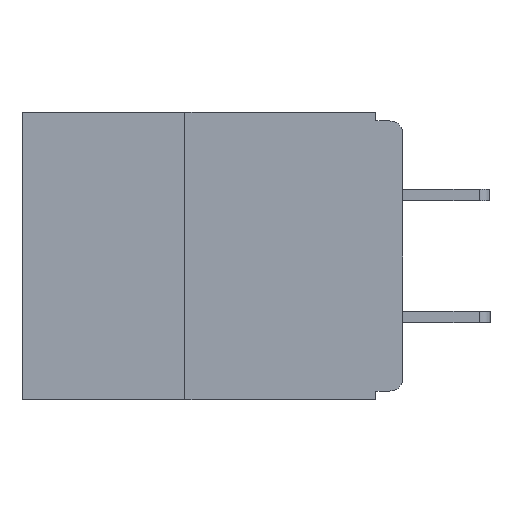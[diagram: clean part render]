
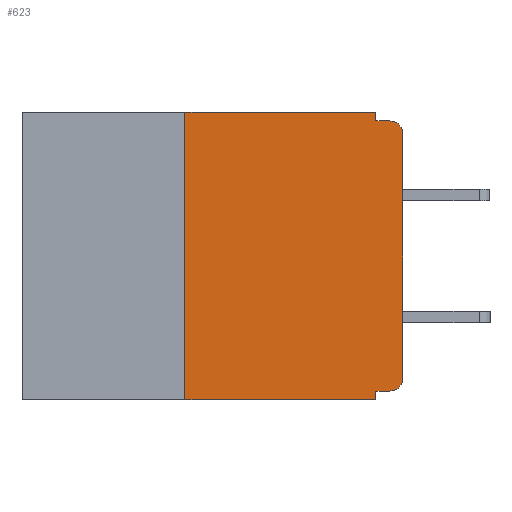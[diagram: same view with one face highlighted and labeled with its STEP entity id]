
A CAD part, left-side view. The second image highlights one B-rep face of the part: STEP entity #623.
In plain terms, the highlighted planar face has unit normal (-1, 0, 0).
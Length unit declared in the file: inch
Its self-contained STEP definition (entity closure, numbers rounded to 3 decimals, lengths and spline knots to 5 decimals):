
#165 = VECTOR ( 'NONE', #5151, 39.37008 ) ;
#623 = ADVANCED_FACE ( 'NONE', ( #1722 ), #1847, .F. ) ;
#680 = VERTEX_POINT ( 'NONE', #10911 ) ;
#707 = EDGE_CURVE ( 'NONE', #10300, #680, #3508, .T. ) ;
#1076 = VERTEX_POINT ( 'NONE', #2092 ) ;
#1090 = LINE ( 'NONE', #6201, #6338 ) ;
#1134 = CARTESIAN_POINT ( 'NONE',  ( 0., 0.015, -0.32 ) ) ;
#1317 = DIRECTION ( 'NONE',  ( 0., 0., 1. ) ) ;
#1501 = AXIS2_PLACEMENT_3D ( 'NONE', #9572, #3896, #10550 ) ;
#1622 = EDGE_CURVE ( 'NONE', #10391, #7050, #1090, .T. ) ;
#1689 = AXIS2_PLACEMENT_3D ( 'NONE', #6691, #3105, #7161 ) ;
#1722 = FACE_OUTER_BOUND ( 'NONE', #4374, .T. ) ;
#1847 = PLANE ( 'NONE',  #7245 ) ;
#1922 = VERTEX_POINT ( 'NONE', #1134 ) ;
#1944 = VERTEX_POINT ( 'NONE', #11863 ) ;
#2092 = CARTESIAN_POINT ( 'NONE',  ( 0., 0.031, -0.32 ) ) ;
#2133 = CARTESIAN_POINT ( 'NONE',  ( 0., 0., 0. ) ) ;
#2451 = DIRECTION ( 'NONE',  ( 0., 0., -1. ) ) ;
#2479 = CARTESIAN_POINT ( 'NONE',  ( 0., 0.015, -0.01 ) ) ;
#2840 = CARTESIAN_POINT ( 'NONE',  ( 0., 0., -0.32 ) ) ;
#2858 = LINE ( 'NONE', #11774, #165 ) ;
#2998 = EDGE_CURVE ( 'NONE', #680, #10391, #6168, .T. ) ;
#3105 = DIRECTION ( 'NONE',  ( -1., 0., 0. ) ) ;
#3428 = CARTESIAN_POINT ( 'NONE',  ( 0., 0.031, -0.33 ) ) ;
#3508 = LINE ( 'NONE', #7914, #8877 ) ;
#3755 = CARTESIAN_POINT ( 'NONE',  ( 0., 0.031, -0.01 ) ) ;
#3896 = DIRECTION ( 'NONE',  ( -1., 0., 0. ) ) ;
#3999 = ORIENTED_EDGE ( 'NONE', *, *, #10636, .T. ) ;
#4087 = EDGE_CURVE ( 'NONE', #1922, #1944, #5985, .T. ) ;
#4145 = DIRECTION ( 'NONE',  ( 1., 0., 0. ) ) ;
#4374 = EDGE_LOOP ( 'NONE', ( #9203, #3999, #7263, #6801, #9052, #5652, #9795, #10099, #8953, #12111 ) ) ;
#4745 = DIRECTION ( 'NONE',  ( 0., 0., -1. ) ) ;
#5121 = VERTEX_POINT ( 'NONE', #2479 ) ;
#5151 = DIRECTION ( 'NONE',  ( 0., -1., 0. ) ) ;
#5175 = CARTESIAN_POINT ( 'NONE',  ( 0., 0., -0.025 ) ) ;
#5315 = CARTESIAN_POINT ( 'NONE',  ( 0., 0.031, 0. ) ) ;
#5644 = EDGE_CURVE ( 'NONE', #7050, #5121, #7927, .T. ) ;
#5652 = ORIENTED_EDGE ( 'NONE', *, *, #707, .F. ) ;
#5707 = CARTESIAN_POINT ( 'NONE',  ( 0., 0.437, 0. ) ) ;
#5985 = CIRCLE ( 'NONE', #1689, 0.015 ) ;
#6168 = LINE ( 'NONE', #11160, #11190 ) ;
#6201 = CARTESIAN_POINT ( 'NONE',  ( 0., 0.031, 0. ) ) ;
#6214 = EDGE_CURVE ( 'NONE', #1944, #10259, #10288, .T. ) ;
#6338 = VECTOR ( 'NONE', #2451, 39.37008 ) ;
#6521 = VECTOR ( 'NONE', #9552, 39.37008 ) ;
#6691 = CARTESIAN_POINT ( 'NONE',  ( 0., 0.015, -0.305 ) ) ;
#6801 = ORIENTED_EDGE ( 'NONE', *, *, #1622, .F. ) ;
#7050 = VERTEX_POINT ( 'NONE', #3755 ) ;
#7161 = DIRECTION ( 'NONE',  ( 0., 0., -1. ) ) ;
#7186 = CARTESIAN_POINT ( 'NONE',  ( 0., 0.031, -0.33 ) ) ;
#7245 = AXIS2_PLACEMENT_3D ( 'NONE', #5707, #4145, #4745 ) ;
#7263 = ORIENTED_EDGE ( 'NONE', *, *, #5644, .F. ) ;
#7585 = EDGE_CURVE ( 'NONE', #1076, #8836, #12124, .T. ) ;
#7763 = VECTOR ( 'NONE', #1317, 39.37008 ) ;
#7836 = DIRECTION ( 'NONE',  ( 0., -1., 0. ) ) ;
#7914 = CARTESIAN_POINT ( 'NONE',  ( 0., 0.25, -0.33 ) ) ;
#7927 = LINE ( 'NONE', #9599, #9553 ) ;
#8482 = EDGE_CURVE ( 'NONE', #1922, #1076, #8754, .T. ) ;
#8754 = LINE ( 'NONE', #2840, #6521 ) ;
#8836 = VERTEX_POINT ( 'NONE', #7186 ) ;
#8877 = VECTOR ( 'NONE', #11070, 39.37008 ) ;
#8953 = ORIENTED_EDGE ( 'NONE', *, *, #8482, .F. ) ;
#9052 = ORIENTED_EDGE ( 'NONE', *, *, #2998, .F. ) ;
#9203 = ORIENTED_EDGE ( 'NONE', *, *, #6214, .T. ) ;
#9437 = CIRCLE ( 'NONE', #1501, 0.015 ) ;
#9552 = DIRECTION ( 'NONE',  ( 0., 1., 0. ) ) ;
#9553 = VECTOR ( 'NONE', #11049, 39.37008 ) ;
#9572 = CARTESIAN_POINT ( 'NONE',  ( 0., 0.015, -0.025 ) ) ;
#9599 = CARTESIAN_POINT ( 'NONE',  ( 0., 0., -0.01 ) ) ;
#9795 = ORIENTED_EDGE ( 'NONE', *, *, #9894, .T. ) ;
#9894 = EDGE_CURVE ( 'NONE', #10300, #8836, #2858, .T. ) ;
#9976 = CARTESIAN_POINT ( 'NONE',  ( 0., 0.25, -0.33 ) ) ;
#10092 = DIRECTION ( 'NONE',  ( 0., 0., -1. ) ) ;
#10099 = ORIENTED_EDGE ( 'NONE', *, *, #7585, .F. ) ;
#10259 = VERTEX_POINT ( 'NONE', #5175 ) ;
#10288 = LINE ( 'NONE', #2133, #7763 ) ;
#10300 = VERTEX_POINT ( 'NONE', #9976 ) ;
#10391 = VERTEX_POINT ( 'NONE', #5315 ) ;
#10550 = DIRECTION ( 'NONE',  ( 0., 0., -1. ) ) ;
#10636 = EDGE_CURVE ( 'NONE', #10259, #5121, #9437, .T. ) ;
#10911 = CARTESIAN_POINT ( 'NONE',  ( 0., 0.25, 0. ) ) ;
#11049 = DIRECTION ( 'NONE',  ( 0., -1., 0. ) ) ;
#11070 = DIRECTION ( 'NONE',  ( 0., 0., 1. ) ) ;
#11160 = CARTESIAN_POINT ( 'NONE',  ( 0., 0.437, 0. ) ) ;
#11190 = VECTOR ( 'NONE', #7836, 39.37008 ) ;
#11774 = CARTESIAN_POINT ( 'NONE',  ( 0., 0.437, -0.33 ) ) ;
#11851 = VECTOR ( 'NONE', #10092, 39.37008 ) ;
#11863 = CARTESIAN_POINT ( 'NONE',  ( 0., 0., -0.305 ) ) ;
#12111 = ORIENTED_EDGE ( 'NONE', *, *, #4087, .T. ) ;
#12124 = LINE ( 'NONE', #3428, #11851 ) ;
